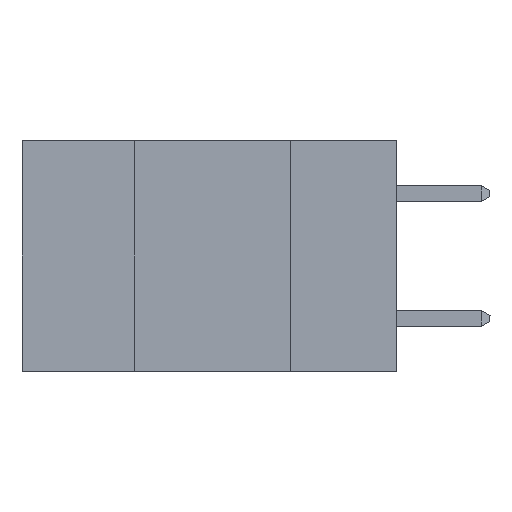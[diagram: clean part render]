
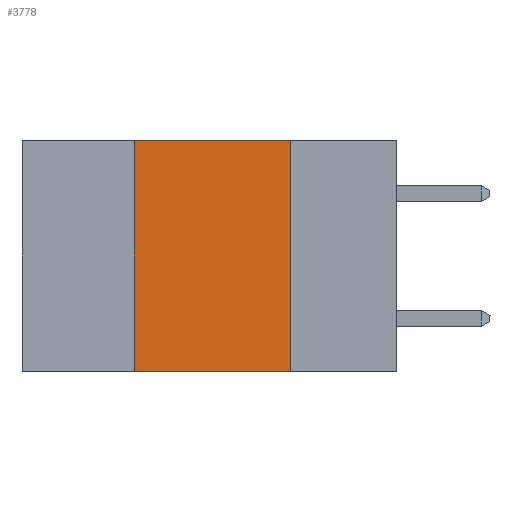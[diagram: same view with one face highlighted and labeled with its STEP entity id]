
A CAD part, left-side view. The second image highlights one B-rep face of the part: STEP entity #3778.
In plain terms, the highlighted planar face has unit normal (-1, 0, 0).
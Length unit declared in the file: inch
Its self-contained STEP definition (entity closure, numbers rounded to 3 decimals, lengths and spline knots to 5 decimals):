
#92 = CARTESIAN_POINT ( 'NONE',  ( 0., 0.42, 0. ) ) ;
#1516 = FACE_OUTER_BOUND ( 'NONE', #3011, .T. ) ;
#2053 = EDGE_CURVE ( 'NONE', #11874, #11225, #10188, .T. ) ;
#2333 = EDGE_CURVE ( 'NONE', #10445, #7849, #5453, .T. ) ;
#2622 = VECTOR ( 'NONE', #11094, 39.37008 ) ;
#2717 = DIRECTION ( 'NONE',  ( 0., 0., -1. ) ) ;
#2804 = DIRECTION ( 'NONE',  ( 0., -1., 0. ) ) ;
#3011 = EDGE_LOOP ( 'NONE', ( #3239, #10876, #3688, #10663 ) ) ;
#3068 = AXIS2_PLACEMENT_3D ( 'NONE', #4788, #8023, #2717 ) ;
#3167 = LINE ( 'NONE', #11398, #10753 ) ;
#3239 = ORIENTED_EDGE ( 'NONE', *, *, #2053, .F. ) ;
#3533 = DIRECTION ( 'NONE',  ( 0., -1., 0. ) ) ;
#3688 = ORIENTED_EDGE ( 'NONE', *, *, #2333, .F. ) ;
#3778 = ADVANCED_FACE ( 'NONE', ( #1516 ), #6927, .F. ) ;
#3806 = CARTESIAN_POINT ( 'NONE',  ( 0., 0.17, 0. ) ) ;
#4044 = CARTESIAN_POINT ( 'NONE',  ( 0., 0.42, -0.37 ) ) ;
#4164 = CARTESIAN_POINT ( 'NONE',  ( 0., 0.17, 0. ) ) ;
#4788 = CARTESIAN_POINT ( 'NONE',  ( 0., 0.6, 0. ) ) ;
#4931 = CARTESIAN_POINT ( 'NONE',  ( 0., 0.17, -0.37 ) ) ;
#5453 = LINE ( 'NONE', #8874, #2622 ) ;
#6420 = VECTOR ( 'NONE', #3533, 39.37008 ) ;
#6927 = PLANE ( 'NONE',  #3068 ) ;
#7849 = VERTEX_POINT ( 'NONE', #92 ) ;
#8023 = DIRECTION ( 'NONE',  ( 1., 0., 0. ) ) ;
#8790 = EDGE_CURVE ( 'NONE', #10445, #11225, #12328, .T. ) ;
#8874 = CARTESIAN_POINT ( 'NONE',  ( 0., 0.42, 0. ) ) ;
#10188 = LINE ( 'NONE', #4164, #11692 ) ;
#10343 = EDGE_CURVE ( 'NONE', #7849, #11874, #3167, .T. ) ;
#10445 = VERTEX_POINT ( 'NONE', #4044 ) ;
#10549 = DIRECTION ( 'NONE',  ( 0., 0., -1. ) ) ;
#10663 = ORIENTED_EDGE ( 'NONE', *, *, #8790, .T. ) ;
#10753 = VECTOR ( 'NONE', #2804, 39.37008 ) ;
#10876 = ORIENTED_EDGE ( 'NONE', *, *, #10343, .F. ) ;
#11094 = DIRECTION ( 'NONE',  ( 0., 0., 1. ) ) ;
#11225 = VERTEX_POINT ( 'NONE', #4931 ) ;
#11398 = CARTESIAN_POINT ( 'NONE',  ( 0., 0.6, 0. ) ) ;
#11692 = VECTOR ( 'NONE', #10549, 39.37008 ) ;
#11874 = VERTEX_POINT ( 'NONE', #3806 ) ;
#12060 = CARTESIAN_POINT ( 'NONE',  ( 0., 0.6, -0.37 ) ) ;
#12328 = LINE ( 'NONE', #12060, #6420 ) ;
